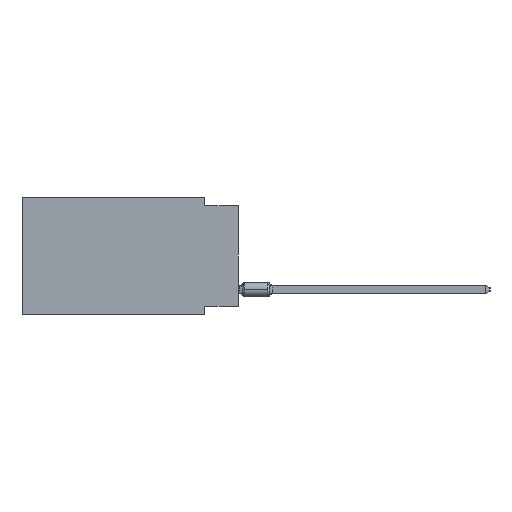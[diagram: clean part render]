
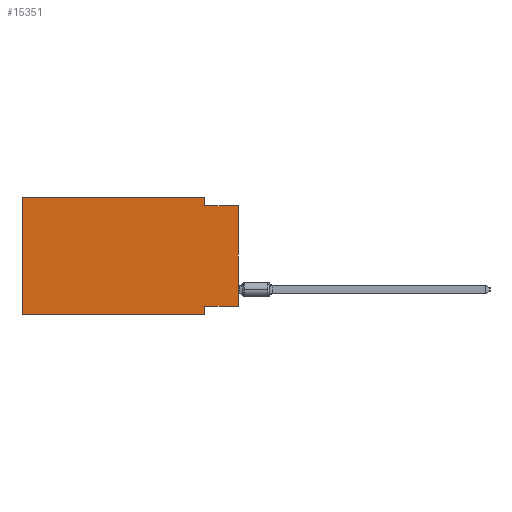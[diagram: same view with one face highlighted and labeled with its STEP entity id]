
A CAD part, left-side view. The second image highlights one B-rep face of the part: STEP entity #15351.
In plain terms, the highlighted planar face has unit normal (-1, 0, 0).
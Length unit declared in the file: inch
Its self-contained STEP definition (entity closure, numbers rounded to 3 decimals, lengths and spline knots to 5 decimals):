
#33 = CARTESIAN_POINT ( 'NONE',  ( 0., 0.645, -0.35 ) ) ;
#464 = CARTESIAN_POINT ( 'NONE',  ( 0., 0.645, -0.35 ) ) ;
#656 = LINE ( 'NONE', #3173, #22434 ) ;
#756 = DIRECTION ( 'NONE',  ( 0., 0., -1. ) ) ;
#1478 = ORIENTED_EDGE ( 'NONE', *, *, #5572, .F. ) ;
#1641 = DIRECTION ( 'NONE',  ( 0., 0., 1. ) ) ;
#1886 = ORIENTED_EDGE ( 'NONE', *, *, #15842, .F. ) ;
#2116 = VECTOR ( 'NONE', #32854, 39.37008 ) ;
#2302 = DIRECTION ( 'NONE',  ( 0., 0., -1. ) ) ;
#2489 = LINE ( 'NONE', #31968, #17567 ) ;
#3173 = CARTESIAN_POINT ( 'NONE',  ( 0., 0.645, 0. ) ) ;
#3622 = VERTEX_POINT ( 'NONE', #464 ) ;
#4442 = LINE ( 'NONE', #34464, #13918 ) ;
#5026 = VERTEX_POINT ( 'NONE', #34216 ) ;
#5572 = EDGE_CURVE ( 'NONE', #3622, #22103, #13697, .T. ) ;
#5871 = DIRECTION ( 'NONE',  ( 0., -1., 0. ) ) ;
#6187 = DIRECTION ( 'NONE',  ( 0., -1., 0. ) ) ;
#6325 = DIRECTION ( 'NONE',  ( 0., 0., -1. ) ) ;
#6734 = CARTESIAN_POINT ( 'NONE',  ( 0., 0., -0.025 ) ) ;
#6811 = ORIENTED_EDGE ( 'NONE', *, *, #24526, .T. ) ;
#7084 = AXIS2_PLACEMENT_3D ( 'NONE', #19955, #25114, #756 ) ;
#7475 = VERTEX_POINT ( 'NONE', #17260 ) ;
#7633 = DIRECTION ( 'NONE',  ( 0., 1., 0. ) ) ;
#8338 = EDGE_CURVE ( 'NONE', #28009, #11166, #14356, .T. ) ;
#8678 = ORIENTED_EDGE ( 'NONE', *, *, #16309, .F. ) ;
#8714 = CARTESIAN_POINT ( 'NONE',  ( 0., 0., -0.025 ) ) ;
#9106 = PLANE ( 'NONE',  #7084 ) ;
#9823 = VERTEX_POINT ( 'NONE', #6734 ) ;
#11166 = VERTEX_POINT ( 'NONE', #25007 ) ;
#11789 = FACE_OUTER_BOUND ( 'NONE', #17445, .T. ) ;
#11902 = VECTOR ( 'NONE', #6325, 39.37008 ) ;
#12419 = EDGE_CURVE ( 'NONE', #24145, #5026, #2489, .T. ) ;
#13697 = LINE ( 'NONE', #19541, #2116 ) ;
#13918 = VECTOR ( 'NONE', #7633, 39.37008 ) ;
#14356 = LINE ( 'NONE', #33346, #11902 ) ;
#15351 = ADVANCED_FACE ( 'NONE', ( #11789 ), #9106, .F. ) ;
#15842 = EDGE_CURVE ( 'NONE', #7475, #28009, #4442, .T. ) ;
#16309 = EDGE_CURVE ( 'NONE', #22103, #24145, #656, .T. ) ;
#17260 = CARTESIAN_POINT ( 'NONE',  ( 0., 0., -0.325 ) ) ;
#17445 = EDGE_LOOP ( 'NONE', ( #27516, #29783, #34154, #8678, #1478, #6811, #28932, #1886 ) ) ;
#17527 = EDGE_CURVE ( 'NONE', #5026, #9823, #21712, .T. ) ;
#17567 = VECTOR ( 'NONE', #2302, 39.37008 ) ;
#19010 = VECTOR ( 'NONE', #5871, 39.37008 ) ;
#19541 = CARTESIAN_POINT ( 'NONE',  ( 0., 0.645, 0. ) ) ;
#19955 = CARTESIAN_POINT ( 'NONE',  ( 0., 0.645, 0. ) ) ;
#21712 = LINE ( 'NONE', #8714, #19010 ) ;
#22103 = VERTEX_POINT ( 'NONE', #25014 ) ;
#22434 = VECTOR ( 'NONE', #32993, 39.37008 ) ;
#24145 = VERTEX_POINT ( 'NONE', #29946 ) ;
#24526 = EDGE_CURVE ( 'NONE', #3622, #11166, #26537, .T. ) ;
#25007 = CARTESIAN_POINT ( 'NONE',  ( 0., 0.1, -0.35 ) ) ;
#25014 = CARTESIAN_POINT ( 'NONE',  ( 0., 0.645, 0. ) ) ;
#25114 = DIRECTION ( 'NONE',  ( 1., 0., 0. ) ) ;
#25818 = LINE ( 'NONE', #28840, #27910 ) ;
#26537 = LINE ( 'NONE', #33, #27169 ) ;
#27169 = VECTOR ( 'NONE', #6187, 39.37008 ) ;
#27516 = ORIENTED_EDGE ( 'NONE', *, *, #35050, .T. ) ;
#27910 = VECTOR ( 'NONE', #1641, 39.37008 ) ;
#28009 = VERTEX_POINT ( 'NONE', #28108 ) ;
#28108 = CARTESIAN_POINT ( 'NONE',  ( 0., 0.1, -0.325 ) ) ;
#28840 = CARTESIAN_POINT ( 'NONE',  ( 0., 0., 0. ) ) ;
#28932 = ORIENTED_EDGE ( 'NONE', *, *, #8338, .F. ) ;
#29783 = ORIENTED_EDGE ( 'NONE', *, *, #17527, .F. ) ;
#29946 = CARTESIAN_POINT ( 'NONE',  ( 0., 0.1, 0. ) ) ;
#31968 = CARTESIAN_POINT ( 'NONE',  ( 0., 0.1, 0. ) ) ;
#32854 = DIRECTION ( 'NONE',  ( 0., 0., 1. ) ) ;
#32993 = DIRECTION ( 'NONE',  ( 0., -1., 0. ) ) ;
#33346 = CARTESIAN_POINT ( 'NONE',  ( 0., 0.1, -0.35 ) ) ;
#34154 = ORIENTED_EDGE ( 'NONE', *, *, #12419, .F. ) ;
#34216 = CARTESIAN_POINT ( 'NONE',  ( 0., 0.1, -0.025 ) ) ;
#34464 = CARTESIAN_POINT ( 'NONE',  ( 0., 0., -0.325 ) ) ;
#35050 = EDGE_CURVE ( 'NONE', #7475, #9823, #25818, .T. ) ;
